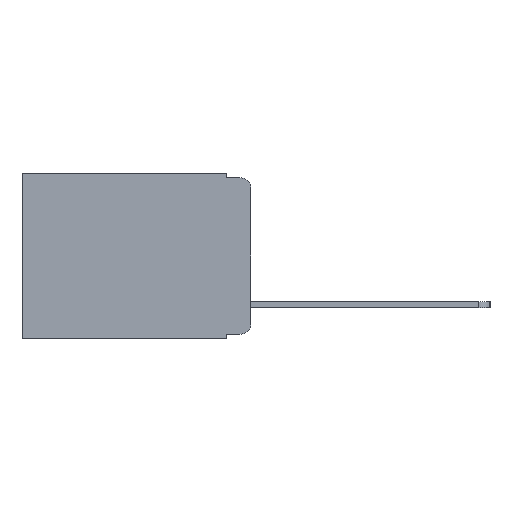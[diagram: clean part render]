
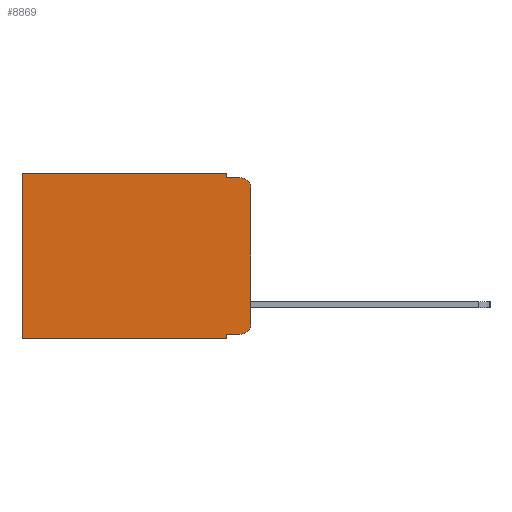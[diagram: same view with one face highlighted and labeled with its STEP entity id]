
A CAD part, left-side view. The second image highlights one B-rep face of the part: STEP entity #8869.
In plain terms, the highlighted planar face has unit normal (-1, 0, 0).
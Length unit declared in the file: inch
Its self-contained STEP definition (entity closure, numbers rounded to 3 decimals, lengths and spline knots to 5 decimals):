
#95 = DIRECTION ( 'NONE',  ( 0., -1., 0. ) ) ;
#510 = LINE ( 'NONE', #9608, #10526 ) ;
#548 = CARTESIAN_POINT ( 'NONE',  ( 0.298, 0., 0. ) ) ;
#756 = ORIENTED_EDGE ( 'NONE', *, *, #4839, .T. ) ;
#826 = FACE_OUTER_BOUND ( 'NONE', #6382, .T. ) ;
#856 = DIRECTION ( 'NONE',  ( 0., 0., -1. ) ) ;
#966 = ORIENTED_EDGE ( 'NONE', *, *, #7321, .T. ) ;
#978 = VECTOR ( 'NONE', #4474, 39.37008 ) ;
#1027 = DIRECTION ( 'NONE',  ( 0., 0., -1. ) ) ;
#1095 = VERTEX_POINT ( 'NONE', #5830 ) ;
#1125 = CARTESIAN_POINT ( 'NONE',  ( 0.298, 0.02, -0.03 ) ) ;
#1164 = VERTEX_POINT ( 'NONE', #1396 ) ;
#1396 = CARTESIAN_POINT ( 'NONE',  ( 0.298, 0.473, -0.343 ) ) ;
#1993 = ORIENTED_EDGE ( 'NONE', *, *, #7287, .T. ) ;
#2047 = CARTESIAN_POINT ( 'NONE',  ( 0.298, 0.051, -0.343 ) ) ;
#2052 = LINE ( 'NONE', #7069, #6858 ) ;
#2216 = DIRECTION ( 'NONE',  ( 0., 0., -1. ) ) ;
#2298 = CARTESIAN_POINT ( 'NONE',  ( 0.298, 0.02, -0.313 ) ) ;
#2378 = VECTOR ( 'NONE', #95, 39.37008 ) ;
#3017 = AXIS2_PLACEMENT_3D ( 'NONE', #1125, #7876, #2216 ) ;
#3131 = LINE ( 'NONE', #6921, #5443 ) ;
#3166 = CARTESIAN_POINT ( 'NONE',  ( 0.298, 0.051, -0.01 ) ) ;
#3205 = DIRECTION ( 'NONE',  ( 0., -1., 0. ) ) ;
#3292 = DIRECTION ( 'NONE',  ( 0., 0., -1. ) ) ;
#3328 = DIRECTION ( 'NONE',  ( 0., 0., -1. ) ) ;
#3740 = VERTEX_POINT ( 'NONE', #8358 ) ;
#4090 = CARTESIAN_POINT ( 'NONE',  ( 0.298, 0.473, 0. ) ) ;
#4287 = AXIS2_PLACEMENT_3D ( 'NONE', #2298, #8866, #3292 ) ;
#4474 = DIRECTION ( 'NONE',  ( 0., 1., 0. ) ) ;
#4529 = VERTEX_POINT ( 'NONE', #2047 ) ;
#4657 = VERTEX_POINT ( 'NONE', #8289 ) ;
#4746 = ORIENTED_EDGE ( 'NONE', *, *, #7359, .F. ) ;
#4839 = EDGE_CURVE ( 'NONE', #11417, #8272, #10854, .T. ) ;
#4874 = CARTESIAN_POINT ( 'NONE',  ( 0.298, 0., 0. ) ) ;
#5443 = VECTOR ( 'NONE', #8740, 39.37008 ) ;
#5612 = VECTOR ( 'NONE', #3205, 39.37008 ) ;
#5830 = CARTESIAN_POINT ( 'NONE',  ( 0.298, 0.02, -0.333 ) ) ;
#5906 = CIRCLE ( 'NONE', #3017, 0.02 ) ;
#5934 = VERTEX_POINT ( 'NONE', #9856 ) ;
#6030 = CARTESIAN_POINT ( 'NONE',  ( 0.298, 0., 0. ) ) ;
#6104 = DIRECTION ( 'NONE',  ( 0., 0., -1. ) ) ;
#6312 = ORIENTED_EDGE ( 'NONE', *, *, #7236, .F. ) ;
#6346 = VERTEX_POINT ( 'NONE', #8695 ) ;
#6382 = EDGE_LOOP ( 'NONE', ( #6312, #8035, #8896, #4746, #756, #1993, #8912, #6810, #966, #10848 ) ) ;
#6762 = DIRECTION ( 'NONE',  ( 1., 0., 0. ) ) ;
#6810 = ORIENTED_EDGE ( 'NONE', *, *, #7298, .F. ) ;
#6858 = VECTOR ( 'NONE', #3328, 39.37008 ) ;
#6921 = CARTESIAN_POINT ( 'NONE',  ( 0.298, 0., -0.343 ) ) ;
#6986 = DIRECTION ( 'NONE',  ( 0., 0., -1. ) ) ;
#7069 = CARTESIAN_POINT ( 'NONE',  ( 0.298, 0.051, 0. ) ) ;
#7236 = EDGE_CURVE ( 'NONE', #4657, #3740, #11024, .T. ) ;
#7276 = EDGE_CURVE ( 'NONE', #4657, #11181, #5906, .T. ) ;
#7279 = EDGE_CURVE ( 'NONE', #6346, #11181, #8003, .T. ) ;
#7287 = EDGE_CURVE ( 'NONE', #8272, #1164, #510, .T. ) ;
#7298 = EDGE_CURVE ( 'NONE', #5934, #4529, #10245, .T. ) ;
#7317 = EDGE_CURVE ( 'NONE', #1095, #3740, #7429, .T. ) ;
#7321 = EDGE_CURVE ( 'NONE', #5934, #1095, #9725, .T. ) ;
#7359 = EDGE_CURVE ( 'NONE', #11417, #6346, #2052, .T. ) ;
#7429 = CIRCLE ( 'NONE', #4287, 0.02 ) ;
#7876 = DIRECTION ( 'NONE',  ( -1., 0., 0. ) ) ;
#7967 = CARTESIAN_POINT ( 'NONE',  ( 0.298, 0.051, 0. ) ) ;
#7970 = CARTESIAN_POINT ( 'NONE',  ( 0.298, 0.051, -0.333 ) ) ;
#8003 = LINE ( 'NONE', #3166, #5612 ) ;
#8035 = ORIENTED_EDGE ( 'NONE', *, *, #7276, .T. ) ;
#8064 = EDGE_CURVE ( 'NONE', #4529, #1164, #3131, .T. ) ;
#8272 = VERTEX_POINT ( 'NONE', #4090 ) ;
#8289 = CARTESIAN_POINT ( 'NONE',  ( 0.298, 0., -0.03 ) ) ;
#8358 = CARTESIAN_POINT ( 'NONE',  ( 0.298, 0., -0.313 ) ) ;
#8584 = AXIS2_PLACEMENT_3D ( 'NONE', #4874, #6762, #856 ) ;
#8695 = CARTESIAN_POINT ( 'NONE',  ( 0.298, 0.051, -0.01 ) ) ;
#8740 = DIRECTION ( 'NONE',  ( 0., 1., 0. ) ) ;
#8792 = CARTESIAN_POINT ( 'NONE',  ( 0.298, 0.051, 0. ) ) ;
#8837 = VECTOR ( 'NONE', #1027, 39.37008 ) ;
#8866 = DIRECTION ( 'NONE',  ( -1., 0., 0. ) ) ;
#8869 = ADVANCED_FACE ( 'NONE', ( #826 ), #9358, .F. ) ;
#8896 = ORIENTED_EDGE ( 'NONE', *, *, #7279, .F. ) ;
#8912 = ORIENTED_EDGE ( 'NONE', *, *, #8064, .F. ) ;
#9346 = CARTESIAN_POINT ( 'NONE',  ( 0.298, 0.02, -0.01 ) ) ;
#9358 = PLANE ( 'NONE',  #8584 ) ;
#9608 = CARTESIAN_POINT ( 'NONE',  ( 0.298, 0.473, 0. ) ) ;
#9725 = LINE ( 'NONE', #7970, #2378 ) ;
#9856 = CARTESIAN_POINT ( 'NONE',  ( 0.298, 0.051, -0.333 ) ) ;
#9984 = VECTOR ( 'NONE', #6104, 39.37008 ) ;
#10245 = LINE ( 'NONE', #8792, #9984 ) ;
#10526 = VECTOR ( 'NONE', #6986, 39.37008 ) ;
#10848 = ORIENTED_EDGE ( 'NONE', *, *, #7317, .T. ) ;
#10854 = LINE ( 'NONE', #548, #978 ) ;
#11024 = LINE ( 'NONE', #6030, #8837 ) ;
#11181 = VERTEX_POINT ( 'NONE', #9346 ) ;
#11417 = VERTEX_POINT ( 'NONE', #7967 ) ;
